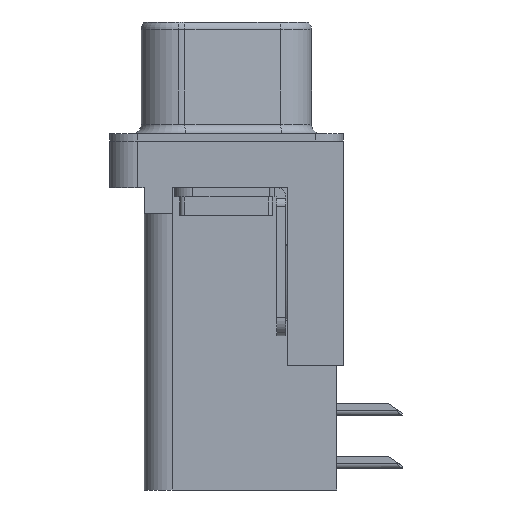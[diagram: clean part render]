
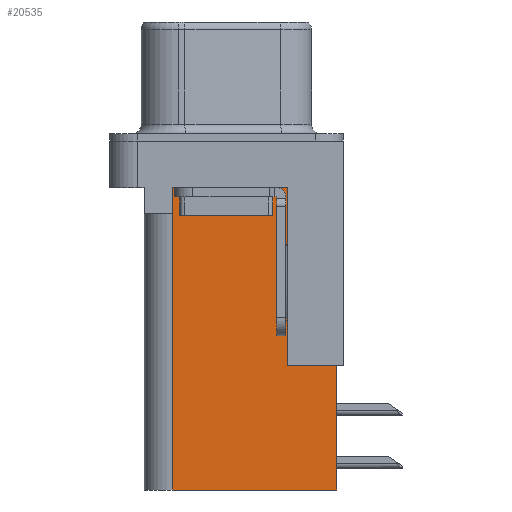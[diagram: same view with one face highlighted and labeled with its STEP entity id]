
A CAD part, left-side view. The second image highlights one B-rep face of the part: STEP entity #20535.
In plain terms, the highlighted planar face has unit normal (-1, 0, 0).
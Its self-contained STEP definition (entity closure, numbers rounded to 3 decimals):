
#297 = DIRECTION ( 'NONE',  ( 0., 0., 1. ) ) ;
#560 = DIRECTION ( 'NONE',  ( 1., 0., 0. ) ) ;
#727 = FACE_OUTER_BOUND ( 'NONE', #2561, .T. ) ;
#1403 = EDGE_CURVE ( 'NONE', #17705, #11028, #1582, .T. ) ;
#1582 = LINE ( 'NONE', #8665, #1640 ) ;
#1640 = VECTOR ( 'NONE', #18075, 1000. ) ;
#1863 = CARTESIAN_POINT ( 'NONE',  ( 3.765, -6.295, -12.05 ) ) ;
#1865 = CARTESIAN_POINT ( 'NONE',  ( 3.765, -3.295, -2.5 ) ) ;
#1980 = CARTESIAN_POINT ( 'NONE',  ( 3.765, -3.295, -18.76 ) ) ;
#2153 = EDGE_CURVE ( 'NONE', #11944, #17705, #11171, .T. ) ;
#2276 = EDGE_CURVE ( 'NONE', #11944, #9111, #8096, .T. ) ;
#2312 = EDGE_CURVE ( 'NONE', #9111, #10334, #7354, .T. ) ;
#2333 = CARTESIAN_POINT ( 'NONE',  ( 3.765, -5.925, -18.76 ) ) ;
#2561 = EDGE_LOOP ( 'NONE', ( #5341, #19787, #13093, #2864, #7310, #11752, #2660, #11951 ) ) ;
#2660 = ORIENTED_EDGE ( 'NONE', *, *, #2276, .T. ) ;
#2864 = ORIENTED_EDGE ( 'NONE', *, *, #19922, .F. ) ;
#2980 = VECTOR ( 'NONE', #297, 1000. ) ;
#2998 = LINE ( 'NONE', #10048, #2980 ) ;
#4807 = EDGE_CURVE ( 'NONE', #10334, #15734, #11091, .T. ) ;
#5341 = ORIENTED_EDGE ( 'NONE', *, *, #4807, .T. ) ;
#6239 = VERTEX_POINT ( 'NONE', #11086 ) ;
#6406 = VECTOR ( 'NONE', #9300, 1000. ) ;
#6593 = LINE ( 'NONE', #7645, #6406 ) ;
#6689 = DIRECTION ( 'NONE',  ( 0., 1., 0. ) ) ;
#7310 = ORIENTED_EDGE ( 'NONE', *, *, #1403, .F. ) ;
#7348 = VECTOR ( 'NONE', #18778, 1000. ) ;
#7354 = LINE ( 'NONE', #1980, #7348 ) ;
#7645 = CARTESIAN_POINT ( 'NONE',  ( 3.765, 0., -3.9 ) ) ;
#7819 = VECTOR ( 'NONE', #6689, 1000. ) ;
#8096 = LINE ( 'NONE', #1863, #7819 ) ;
#8639 = CARTESIAN_POINT ( 'NONE',  ( 3.765, -3.295, -18.76 ) ) ;
#8665 = CARTESIAN_POINT ( 'NONE',  ( 3.765, -3.295, -18.76 ) ) ;
#9111 = VERTEX_POINT ( 'NONE', #12748 ) ;
#9300 = DIRECTION ( 'NONE',  ( 0., 1., 0. ) ) ;
#10048 = CARTESIAN_POINT ( 'NONE',  ( 3.765, 2.925, -18.76 ) ) ;
#10334 = VERTEX_POINT ( 'NONE', #13127 ) ;
#10347 = VECTOR ( 'NONE', #17593, 1000. ) ;
#10713 = DIRECTION ( 'NONE',  ( 0., 0., -1. ) ) ;
#10894 = CARTESIAN_POINT ( 'NONE',  ( 3.765, 2.895, -2.5 ) ) ;
#11028 = VERTEX_POINT ( 'NONE', #20139 ) ;
#11051 = CARTESIAN_POINT ( 'NONE',  ( 3.765, -5.925, -2. ) ) ;
#11086 = CARTESIAN_POINT ( 'NONE',  ( 3.765, 2.895, -3.9 ) ) ;
#11091 = LINE ( 'NONE', #1865, #10347 ) ;
#11171 = LINE ( 'NONE', #11051, #11612 ) ;
#11612 = VECTOR ( 'NONE', #10713, 1000. ) ;
#11752 = ORIENTED_EDGE ( 'NONE', *, *, #2153, .F. ) ;
#11797 = PLANE ( 'NONE',  #16886 ) ;
#11873 = DIRECTION ( 'NONE',  ( 0., 1., 0. ) ) ;
#11925 = CARTESIAN_POINT ( 'NONE',  ( 3.765, 2.895, -3.9 ) ) ;
#11944 = VERTEX_POINT ( 'NONE', #17543 ) ;
#11951 = ORIENTED_EDGE ( 'NONE', *, *, #2312, .T. ) ;
#12314 = VECTOR ( 'NONE', #18296, 1000. ) ;
#12341 = LINE ( 'NONE', #11925, #12314 ) ;
#12748 = CARTESIAN_POINT ( 'NONE',  ( 3.765, -3.295, -12.05 ) ) ;
#13093 = ORIENTED_EDGE ( 'NONE', *, *, #19107, .T. ) ;
#13127 = CARTESIAN_POINT ( 'NONE',  ( 3.765, -3.295, -2.5 ) ) ;
#14856 = VERTEX_POINT ( 'NONE', #19879 ) ;
#15734 = VERTEX_POINT ( 'NONE', #10894 ) ;
#16886 = AXIS2_PLACEMENT_3D ( 'NONE', #8639, #560, #11873 ) ;
#17218 = EDGE_CURVE ( 'NONE', #15734, #6239, #12341, .T. ) ;
#17543 = CARTESIAN_POINT ( 'NONE',  ( 3.765, -5.925, -12.05 ) ) ;
#17593 = DIRECTION ( 'NONE',  ( 0., 1., 0. ) ) ;
#17705 = VERTEX_POINT ( 'NONE', #2333 ) ;
#18075 = DIRECTION ( 'NONE',  ( 0., 1., 0. ) ) ;
#18296 = DIRECTION ( 'NONE',  ( 0., 0., -1. ) ) ;
#18778 = DIRECTION ( 'NONE',  ( 0., 0., 1. ) ) ;
#19107 = EDGE_CURVE ( 'NONE', #6239, #14856, #6593, .T. ) ;
#19787 = ORIENTED_EDGE ( 'NONE', *, *, #17218, .T. ) ;
#19879 = CARTESIAN_POINT ( 'NONE',  ( 3.765, 2.925, -3.9 ) ) ;
#19922 = EDGE_CURVE ( 'NONE', #11028, #14856, #2998, .T. ) ;
#20139 = CARTESIAN_POINT ( 'NONE',  ( 3.765, 2.925, -18.76 ) ) ;
#20535 = ADVANCED_FACE ( 'NONE', ( #727 ), #11797, .F. ) ;
